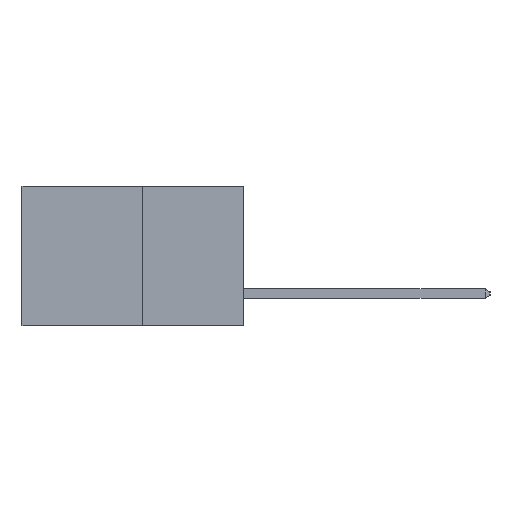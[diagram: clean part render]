
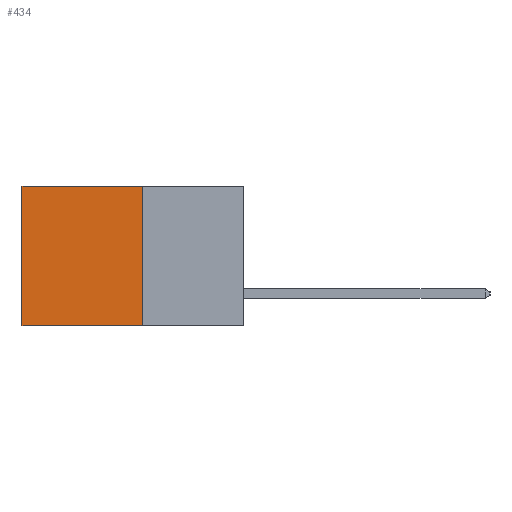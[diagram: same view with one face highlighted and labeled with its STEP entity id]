
A CAD part, left-side view. The second image highlights one B-rep face of the part: STEP entity #434.
In plain terms, the highlighted planar face has unit normal (-1, 0, 0).
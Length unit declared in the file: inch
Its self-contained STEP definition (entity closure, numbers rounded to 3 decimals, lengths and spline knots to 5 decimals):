
#369 = DIRECTION ( 'NONE',  ( 1., 0., 0. ) ) ;
#380 = DIRECTION ( 'NONE',  ( 0., 0., -1. ) ) ;
#434 = ADVANCED_FACE ( 'NONE', ( #7143 ), #7323, .F. ) ;
#667 = ORIENTED_EDGE ( 'NONE', *, *, #1863, .F. ) ;
#701 = CARTESIAN_POINT ( 'NONE',  ( 0.277, 0.27, 0. ) ) ;
#962 = AXIS2_PLACEMENT_3D ( 'NONE', #2467, #369, #380 ) ;
#1441 = EDGE_CURVE ( 'NONE', #1722, #10099, #4405, .T. ) ;
#1722 = VERTEX_POINT ( 'NONE', #9391 ) ;
#1844 = VECTOR ( 'NONE', #5251, 39.37008 ) ;
#1863 = EDGE_CURVE ( 'NONE', #2177, #10099, #8783, .T. ) ;
#2177 = VERTEX_POINT ( 'NONE', #8962 ) ;
#2225 = LINE ( 'NONE', #2917, #8885 ) ;
#2467 = CARTESIAN_POINT ( 'NONE',  ( 0.277, 0.27, -0.37 ) ) ;
#2700 = ORIENTED_EDGE ( 'NONE', *, *, #1441, .T. ) ;
#2917 = CARTESIAN_POINT ( 'NONE',  ( 0.277, 0.27, -0.37 ) ) ;
#3836 = LINE ( 'NONE', #701, #10161 ) ;
#3910 = CARTESIAN_POINT ( 'NONE',  ( 0.277, 0.59, -0.37 ) ) ;
#4198 = ORIENTED_EDGE ( 'NONE', *, *, #9683, .T. ) ;
#4225 = DIRECTION ( 'NONE',  ( 0., 1., 0. ) ) ;
#4405 = LINE ( 'NONE', #5775, #1844 ) ;
#4745 = CARTESIAN_POINT ( 'NONE',  ( 0.277, 0.27, -0.37 ) ) ;
#5251 = DIRECTION ( 'NONE',  ( 0., 0., -1. ) ) ;
#5775 = CARTESIAN_POINT ( 'NONE',  ( 0.277, 0.59, -0.37 ) ) ;
#6338 = VERTEX_POINT ( 'NONE', #10150 ) ;
#6590 = ORIENTED_EDGE ( 'NONE', *, *, #9389, .F. ) ;
#7143 = FACE_OUTER_BOUND ( 'NONE', #9229, .T. ) ;
#7323 = PLANE ( 'NONE',  #962 ) ;
#7921 = DIRECTION ( 'NONE',  ( 0., 0., -1. ) ) ;
#8783 = LINE ( 'NONE', #4745, #10698 ) ;
#8885 = VECTOR ( 'NONE', #7921, 39.37008 ) ;
#8962 = CARTESIAN_POINT ( 'NONE',  ( 0.277, 0.27, -0.37 ) ) ;
#9080 = DIRECTION ( 'NONE',  ( 0., 1., 0. ) ) ;
#9229 = EDGE_LOOP ( 'NONE', ( #2700, #667, #6590, #4198 ) ) ;
#9389 = EDGE_CURVE ( 'NONE', #6338, #2177, #2225, .T. ) ;
#9391 = CARTESIAN_POINT ( 'NONE',  ( 0.277, 0.59, 0. ) ) ;
#9683 = EDGE_CURVE ( 'NONE', #6338, #1722, #3836, .T. ) ;
#10099 = VERTEX_POINT ( 'NONE', #3910 ) ;
#10150 = CARTESIAN_POINT ( 'NONE',  ( 0.277, 0.27, 0. ) ) ;
#10161 = VECTOR ( 'NONE', #9080, 39.37008 ) ;
#10698 = VECTOR ( 'NONE', #4225, 39.37008 ) ;
